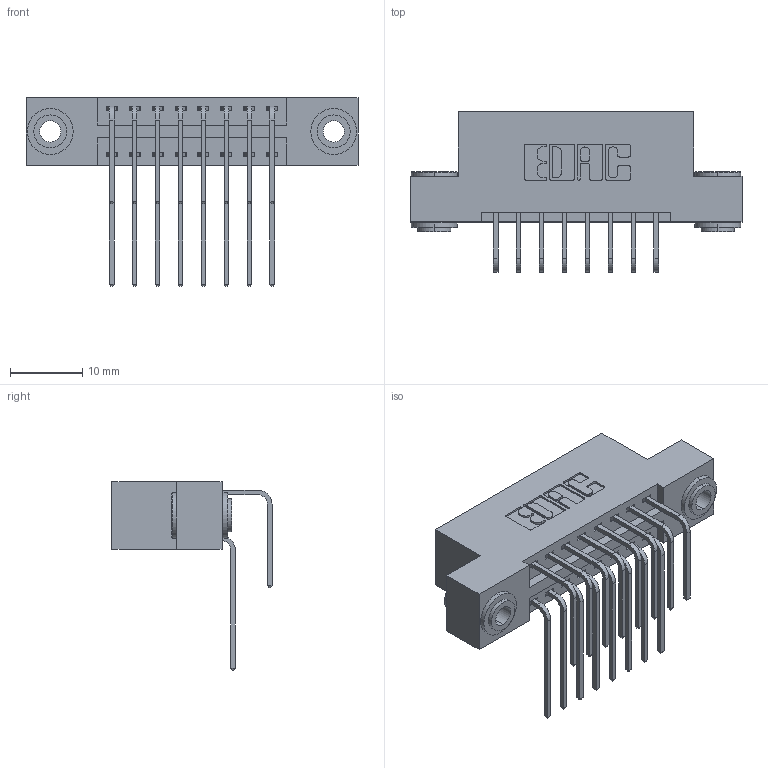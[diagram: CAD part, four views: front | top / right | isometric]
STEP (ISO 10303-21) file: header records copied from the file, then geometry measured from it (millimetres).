
FILE_DESCRIPTION (( 'STEP AP203' ), '1' );
FILE_NAME ('396-016-558-203.STEP', '2019-11-02T13:54:10', ( '' ), ( '' ), 'SwSTEP 2.0', 'SolidWorks 2016', '' );
FILE_SCHEMA (( 'CONFIG_CONTROL_DESIGN' ));
Length unit declared in the file: inch
Products named in the file (5): 396-016-558-203; 346 Part_Flush Mounting Lugs - 0.156 Dia-TH; 345-292-001_558 559 Tail - 1; 345-292-001_558 Tail - 2; 345-250-002_345-250-002-102
Assembly tree (19 placements, depth 2):
  396-016-558-203
    346 Part_Flush Mounting Lugs - 0.156 Dia-TH
    345-292-001_558 559 Tail - 1  x8
    345-292-001_558 Tail - 2  x8
    345-250-002_345-250-002-102  x2
Bounding box: 45.97 x 22.16 x 26.16 mm (x, y, z)
Volume: 4330.7 mm3; surface area: 6075.4 mm2
Topology: 19 solids, 19 shells, 1024 faces, 2981 edges, 1962 vertices
Faces by surface type: plane 678, cylinder 338, cone 8
Entity records: 12232 total; most frequent: CARTESIAN_POINT 2090, ORIENTED_EDGE 1966, DIRECTION 1897, EDGE_CURVE 983, VECTOR 755, LINE 755, VERTEX_POINT 650, AXIS2_PLACEMENT_3D 571
